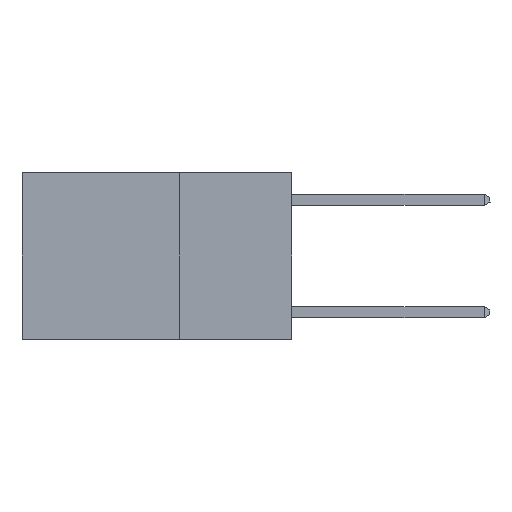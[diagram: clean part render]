
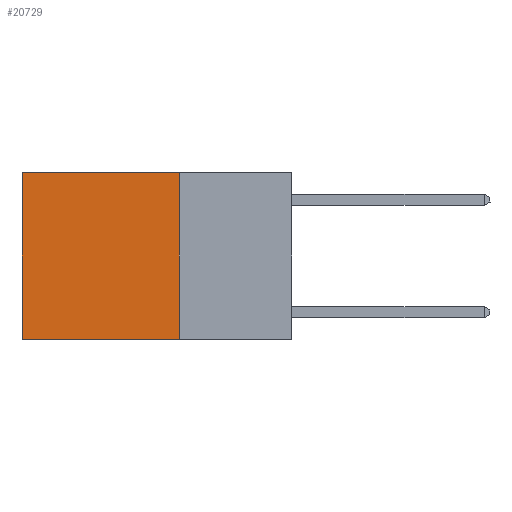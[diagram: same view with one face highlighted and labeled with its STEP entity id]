
A CAD part, left-side view. The second image highlights one B-rep face of the part: STEP entity #20729.
In plain terms, the highlighted planar face has unit normal (-1, 0, 0).
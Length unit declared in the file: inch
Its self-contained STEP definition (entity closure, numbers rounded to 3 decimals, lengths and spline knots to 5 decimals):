
#1180 = DIRECTION ( 'NONE',  ( 0., 0., -1. ) ) ;
#1808 = LINE ( 'NONE', #6150, #14760 ) ;
#2552 = AXIS2_PLACEMENT_3D ( 'NONE', #11647, #23377, #30406 ) ;
#3373 = DIRECTION ( 'NONE',  ( 0., 0., -1. ) ) ;
#4292 = VERTEX_POINT ( 'NONE', #16774 ) ;
#5675 = CARTESIAN_POINT ( 'NONE',  ( 0.2625, 0.25, 0. ) ) ;
#6150 = CARTESIAN_POINT ( 'NONE',  ( 0.2625, 0.6, 0. ) ) ;
#6372 = CARTESIAN_POINT ( 'NONE',  ( 0.2625, 0.25, 0. ) ) ;
#7231 = CARTESIAN_POINT ( 'NONE',  ( 0.2625, 0.6, -0.37 ) ) ;
#7867 = EDGE_LOOP ( 'NONE', ( #23364, #28172, #14401, #11953 ) ) ;
#8712 = PLANE ( 'NONE',  #2552 ) ;
#10518 = VECTOR ( 'NONE', #3373, 39.37008 ) ;
#11021 = DIRECTION ( 'NONE',  ( 0., 1., 0. ) ) ;
#11647 = CARTESIAN_POINT ( 'NONE',  ( 0.2625, 0.25, 0. ) ) ;
#11953 = ORIENTED_EDGE ( 'NONE', *, *, #22996, .T. ) ;
#13227 = LINE ( 'NONE', #15401, #25939 ) ;
#14401 = ORIENTED_EDGE ( 'NONE', *, *, #21969, .F. ) ;
#14760 = VECTOR ( 'NONE', #1180, 39.37008 ) ;
#15401 = CARTESIAN_POINT ( 'NONE',  ( 0.2625, 0.25, -0.37 ) ) ;
#16710 = VERTEX_POINT ( 'NONE', #23303 ) ;
#16774 = CARTESIAN_POINT ( 'NONE',  ( 0.2625, 0.25, 0. ) ) ;
#20357 = VERTEX_POINT ( 'NONE', #21396 ) ;
#20729 = ADVANCED_FACE ( 'NONE', ( #25365 ), #8712, .F. ) ;
#21396 = CARTESIAN_POINT ( 'NONE',  ( 0.2625, 0.6, 0. ) ) ;
#21754 = VERTEX_POINT ( 'NONE', #7231 ) ;
#21969 = EDGE_CURVE ( 'NONE', #4292, #16710, #29113, .T. ) ;
#22996 = EDGE_CURVE ( 'NONE', #4292, #20357, #29956, .T. ) ;
#23303 = CARTESIAN_POINT ( 'NONE',  ( 0.2625, 0.25, -0.37 ) ) ;
#23364 = ORIENTED_EDGE ( 'NONE', *, *, #28455, .T. ) ;
#23377 = DIRECTION ( 'NONE',  ( 1., 0., 0. ) ) ;
#24260 = EDGE_CURVE ( 'NONE', #16710, #21754, #13227, .T. ) ;
#24611 = DIRECTION ( 'NONE',  ( 0., 1., 0. ) ) ;
#25365 = FACE_OUTER_BOUND ( 'NONE', #7867, .T. ) ;
#25939 = VECTOR ( 'NONE', #24611, 39.37008 ) ;
#28172 = ORIENTED_EDGE ( 'NONE', *, *, #24260, .F. ) ;
#28300 = VECTOR ( 'NONE', #11021, 39.37008 ) ;
#28455 = EDGE_CURVE ( 'NONE', #20357, #21754, #1808, .T. ) ;
#29113 = LINE ( 'NONE', #5675, #10518 ) ;
#29956 = LINE ( 'NONE', #6372, #28300 ) ;
#30406 = DIRECTION ( 'NONE',  ( 0., 0., -1. ) ) ;
